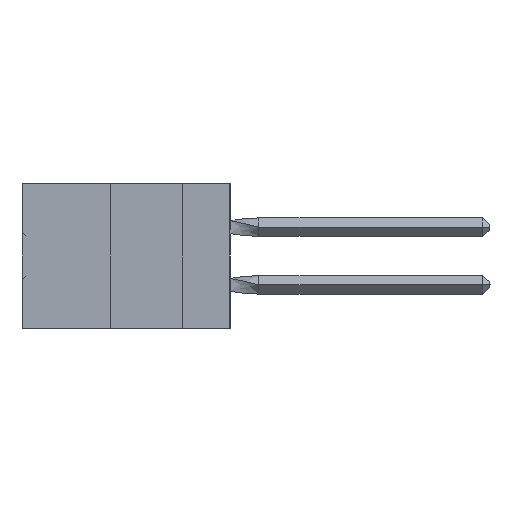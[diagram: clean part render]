
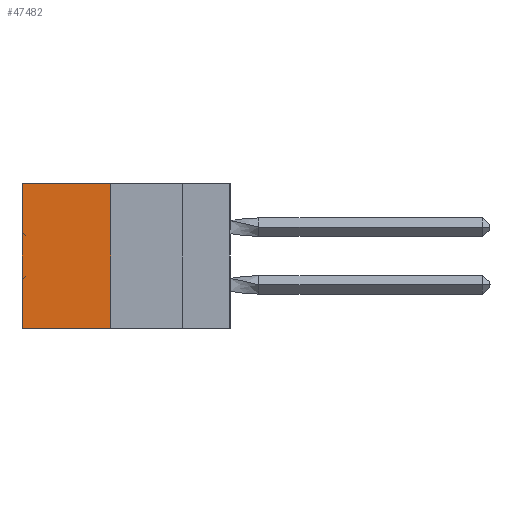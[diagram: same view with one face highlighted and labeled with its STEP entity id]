
A CAD part, left-side view. The second image highlights one B-rep face of the part: STEP entity #47482.
In plain terms, the highlighted planar face has unit normal (-1, 0, 0).
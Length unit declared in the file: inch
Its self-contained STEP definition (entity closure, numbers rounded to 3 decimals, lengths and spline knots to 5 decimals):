
#461 = DIRECTION ( 'NONE',  ( 0., 1., 0. ) ) ;
#1575 = CARTESIAN_POINT ( 'NONE',  ( 0.305, 0.413, -0.5 ) ) ;
#3307 = DIRECTION ( 'NONE',  ( 0., 0., -1. ) ) ;
#3939 = EDGE_CURVE ( 'NONE', #16660, #29375, #26739, .T. ) ;
#5780 = CARTESIAN_POINT ( 'NONE',  ( 0.305, 0.72, -0.5 ) ) ;
#6659 = VECTOR ( 'NONE', #3307, 39.37008 ) ;
#7934 = CARTESIAN_POINT ( 'NONE',  ( 0.305, 0.413, 0. ) ) ;
#8723 = EDGE_CURVE ( 'NONE', #16660, #53452, #35826, .T. ) ;
#8900 = CARTESIAN_POINT ( 'NONE',  ( 0.305, 0.413, 0. ) ) ;
#13313 = VECTOR ( 'NONE', #41144, 39.37008 ) ;
#14384 = LINE ( 'NONE', #48720, #43583 ) ;
#16408 = FACE_OUTER_BOUND ( 'NONE', #28382, .T. ) ;
#16660 = VERTEX_POINT ( 'NONE', #8900 ) ;
#19129 = CARTESIAN_POINT ( 'NONE',  ( 0.305, 0.413, -0.5 ) ) ;
#19236 = ORIENTED_EDGE ( 'NONE', *, *, #8723, .F. ) ;
#21334 = VECTOR ( 'NONE', #461, 39.37008 ) ;
#26111 = EDGE_CURVE ( 'NONE', #53452, #57977, #34050, .T. ) ;
#26739 = LINE ( 'NONE', #7934, #13313 ) ;
#27039 = ORIENTED_EDGE ( 'NONE', *, *, #26111, .F. ) ;
#28382 = EDGE_LOOP ( 'NONE', ( #29323, #27039, #19236, #35396 ) ) ;
#29323 = ORIENTED_EDGE ( 'NONE', *, *, #53981, .T. ) ;
#29375 = VERTEX_POINT ( 'NONE', #47861 ) ;
#32148 = DIRECTION ( 'NONE',  ( 0., 0., -1. ) ) ;
#34050 = LINE ( 'NONE', #19129, #21334 ) ;
#35396 = ORIENTED_EDGE ( 'NONE', *, *, #3939, .T. ) ;
#35826 = LINE ( 'NONE', #35930, #6659 ) ;
#35930 = CARTESIAN_POINT ( 'NONE',  ( 0.305, 0.413, -0.5 ) ) ;
#36966 = DIRECTION ( 'NONE',  ( 1., 0., 0. ) ) ;
#41144 = DIRECTION ( 'NONE',  ( 0., 1., 0. ) ) ;
#43542 = AXIS2_PLACEMENT_3D ( 'NONE', #55650, #36966, #32148 ) ;
#43583 = VECTOR ( 'NONE', #53496, 39.37008 ) ;
#46313 = PLANE ( 'NONE',  #43542 ) ;
#47482 = ADVANCED_FACE ( 'NONE', ( #16408 ), #46313, .F. ) ;
#47861 = CARTESIAN_POINT ( 'NONE',  ( 0.305, 0.72, 0. ) ) ;
#48720 = CARTESIAN_POINT ( 'NONE',  ( 0.305, 0.72, -0.5 ) ) ;
#53452 = VERTEX_POINT ( 'NONE', #1575 ) ;
#53496 = DIRECTION ( 'NONE',  ( 0., 0., -1. ) ) ;
#53981 = EDGE_CURVE ( 'NONE', #29375, #57977, #14384, .T. ) ;
#55650 = CARTESIAN_POINT ( 'NONE',  ( 0.305, 0.413, -0.5 ) ) ;
#57977 = VERTEX_POINT ( 'NONE', #5780 ) ;
